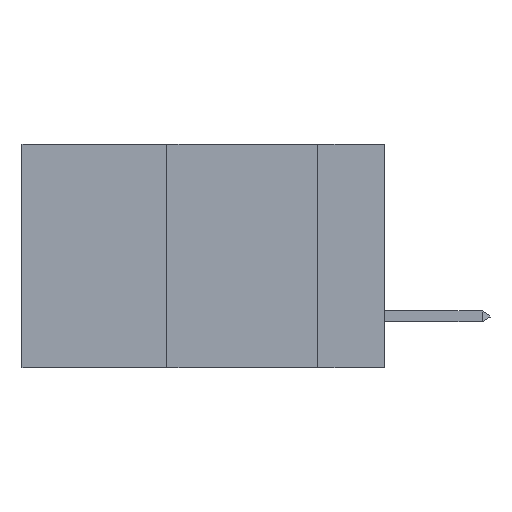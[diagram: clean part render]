
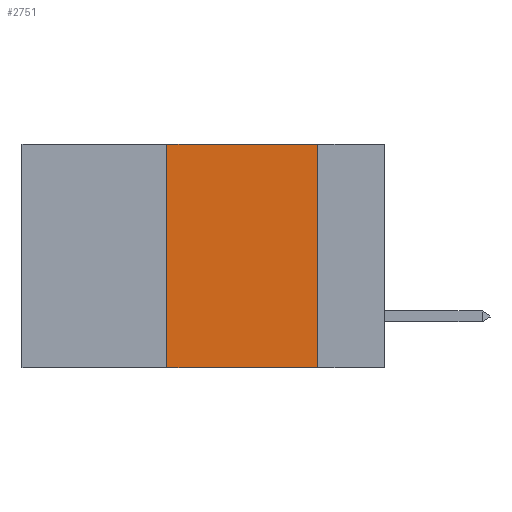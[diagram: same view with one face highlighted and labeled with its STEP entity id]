
A CAD part, left-side view. The second image highlights one B-rep face of the part: STEP entity #2751.
In plain terms, the highlighted planar face has unit normal (-1, 0, 0).
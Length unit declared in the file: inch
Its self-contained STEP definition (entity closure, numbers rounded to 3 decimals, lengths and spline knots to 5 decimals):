
#61 = ORIENTED_EDGE ( 'NONE', *, *, #8523, .F. ) ;
#98 = CARTESIAN_POINT ( 'NONE',  ( 0., 0.11, 0. ) ) ;
#331 = DIRECTION ( 'NONE',  ( 1., 0., 0. ) ) ;
#739 = VERTEX_POINT ( 'NONE', #4468 ) ;
#967 = ORIENTED_EDGE ( 'NONE', *, *, #2942, .F. ) ;
#1566 = LINE ( 'NONE', #6776, #3567 ) ;
#1657 = VERTEX_POINT ( 'NONE', #7751 ) ;
#2162 = VERTEX_POINT ( 'NONE', #7445 ) ;
#2317 = LINE ( 'NONE', #7206, #4285 ) ;
#2751 = ADVANCED_FACE ( 'NONE', ( #6628 ), #8715, .F. ) ;
#2924 = ORIENTED_EDGE ( 'NONE', *, *, #4796, .T. ) ;
#2942 = EDGE_CURVE ( 'NONE', #739, #1657, #3957, .T. ) ;
#3567 = VECTOR ( 'NONE', #6714, 39.37008 ) ;
#3957 = LINE ( 'NONE', #4887, #9020 ) ;
#4100 = DIRECTION ( 'NONE',  ( 0., -1., 0. ) ) ;
#4285 = VECTOR ( 'NONE', #4100, 39.37008 ) ;
#4468 = CARTESIAN_POINT ( 'NONE',  ( 0., 0.36, -0.37 ) ) ;
#4796 = EDGE_CURVE ( 'NONE', #739, #2162, #2317, .T. ) ;
#4887 = CARTESIAN_POINT ( 'NONE',  ( 0., 0.36, 0. ) ) ;
#5476 = DIRECTION ( 'NONE',  ( 0., 0., -1. ) ) ;
#6628 = FACE_OUTER_BOUND ( 'NONE', #8864, .T. ) ;
#6714 = DIRECTION ( 'NONE',  ( 0., -1., 0. ) ) ;
#6762 = AXIS2_PLACEMENT_3D ( 'NONE', #9463, #331, #9434 ) ;
#6776 = CARTESIAN_POINT ( 'NONE',  ( 0., 0.6, 0. ) ) ;
#6827 = LINE ( 'NONE', #8069, #7647 ) ;
#7129 = EDGE_CURVE ( 'NONE', #1657, #9826, #1566, .T. ) ;
#7206 = CARTESIAN_POINT ( 'NONE',  ( 0., 0.6, -0.37 ) ) ;
#7445 = CARTESIAN_POINT ( 'NONE',  ( 0., 0.11, -0.37 ) ) ;
#7647 = VECTOR ( 'NONE', #5476, 39.37008 ) ;
#7751 = CARTESIAN_POINT ( 'NONE',  ( 0., 0.36, 0. ) ) ;
#8069 = CARTESIAN_POINT ( 'NONE',  ( 0., 0.11, 0. ) ) ;
#8523 = EDGE_CURVE ( 'NONE', #9826, #2162, #6827, .T. ) ;
#8715 = PLANE ( 'NONE',  #6762 ) ;
#8864 = EDGE_LOOP ( 'NONE', ( #61, #10458, #967, #2924 ) ) ;
#9020 = VECTOR ( 'NONE', #10622, 39.37008 ) ;
#9434 = DIRECTION ( 'NONE',  ( 0., 0., -1. ) ) ;
#9463 = CARTESIAN_POINT ( 'NONE',  ( 0., 0.6, 0. ) ) ;
#9826 = VERTEX_POINT ( 'NONE', #98 ) ;
#10458 = ORIENTED_EDGE ( 'NONE', *, *, #7129, .F. ) ;
#10622 = DIRECTION ( 'NONE',  ( 0., 0., 1. ) ) ;
